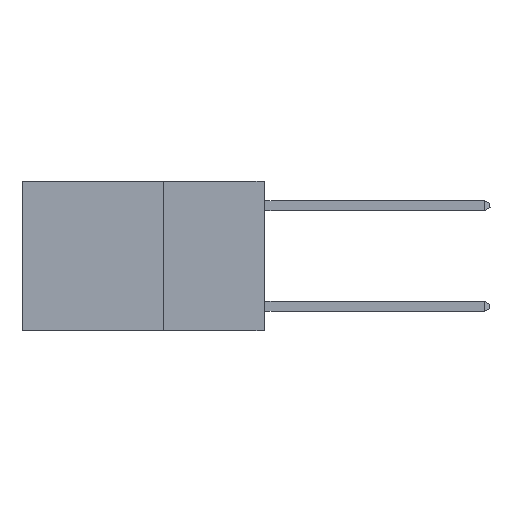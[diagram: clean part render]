
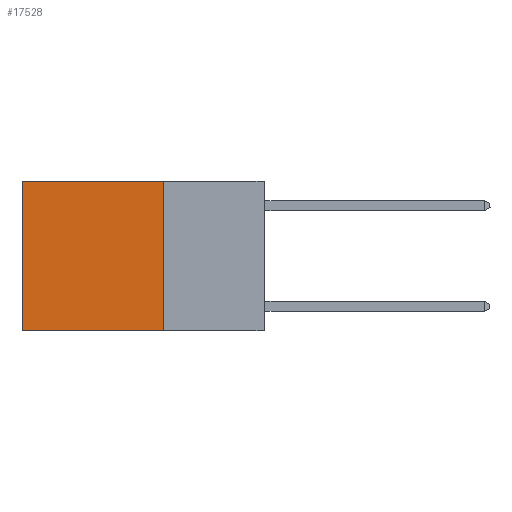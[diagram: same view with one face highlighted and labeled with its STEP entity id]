
A CAD part, left-side view. The second image highlights one B-rep face of the part: STEP entity #17528.
In plain terms, the highlighted planar face has unit normal (-1, 0, 0).
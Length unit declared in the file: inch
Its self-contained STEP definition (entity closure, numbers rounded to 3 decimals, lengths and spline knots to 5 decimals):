
#494 = DIRECTION ( 'NONE',  ( 0., 1., 0. ) ) ;
#1168 = FACE_OUTER_BOUND ( 'NONE', #11827, .T. ) ;
#1943 = EDGE_CURVE ( 'NONE', #18034, #6293, #9952, .T. ) ;
#2007 = CARTESIAN_POINT ( 'NONE',  ( 0.2625, 0.25, 0. ) ) ;
#2605 = DIRECTION ( 'NONE',  ( 1., 0., 0. ) ) ;
#3637 = LINE ( 'NONE', #17984, #12807 ) ;
#5821 = CARTESIAN_POINT ( 'NONE',  ( 0.2625, 0.25, 0. ) ) ;
#6230 = DIRECTION ( 'NONE',  ( 0., 0., -1. ) ) ;
#6293 = VERTEX_POINT ( 'NONE', #15637 ) ;
#7214 = VERTEX_POINT ( 'NONE', #13466 ) ;
#7268 = LINE ( 'NONE', #12769, #22412 ) ;
#9266 = EDGE_CURVE ( 'NONE', #6293, #10761, #21585, .T. ) ;
#9952 = LINE ( 'NONE', #5821, #19855 ) ;
#10431 = ORIENTED_EDGE ( 'NONE', *, *, #9266, .T. ) ;
#10761 = VERTEX_POINT ( 'NONE', #19681 ) ;
#11425 = CARTESIAN_POINT ( 'NONE',  ( 0.2625, 0.25, 0. ) ) ;
#11827 = EDGE_LOOP ( 'NONE', ( #10431, #15646, #11985, #21943 ) ) ;
#11985 = ORIENTED_EDGE ( 'NONE', *, *, #14257, .F. ) ;
#12234 = VECTOR ( 'NONE', #20776, 39.37008 ) ;
#12769 = CARTESIAN_POINT ( 'NONE',  ( 0.2625, 0.25, 0. ) ) ;
#12807 = VECTOR ( 'NONE', #12853, 39.37008 ) ;
#12853 = DIRECTION ( 'NONE',  ( 0., 1., 0. ) ) ;
#13092 = CARTESIAN_POINT ( 'NONE',  ( 0.2625, 0.6, 0. ) ) ;
#13466 = CARTESIAN_POINT ( 'NONE',  ( 0.2625, 0.25, -0.37 ) ) ;
#13933 = EDGE_CURVE ( 'NONE', #7214, #10761, #3637, .T. ) ;
#14257 = EDGE_CURVE ( 'NONE', #18034, #7214, #7268, .T. ) ;
#15108 = DIRECTION ( 'NONE',  ( 0., 0., -1. ) ) ;
#15637 = CARTESIAN_POINT ( 'NONE',  ( 0.2625, 0.6, 0. ) ) ;
#15646 = ORIENTED_EDGE ( 'NONE', *, *, #13933, .F. ) ;
#17528 = ADVANCED_FACE ( 'NONE', ( #1168 ), #22168, .F. ) ;
#17984 = CARTESIAN_POINT ( 'NONE',  ( 0.2625, 0.25, -0.37 ) ) ;
#18034 = VERTEX_POINT ( 'NONE', #2007 ) ;
#19681 = CARTESIAN_POINT ( 'NONE',  ( 0.2625, 0.6, -0.37 ) ) ;
#19855 = VECTOR ( 'NONE', #494, 39.37008 ) ;
#20776 = DIRECTION ( 'NONE',  ( 0., 0., -1. ) ) ;
#21585 = LINE ( 'NONE', #13092, #12234 ) ;
#21943 = ORIENTED_EDGE ( 'NONE', *, *, #1943, .T. ) ;
#22168 = PLANE ( 'NONE',  #22731 ) ;
#22412 = VECTOR ( 'NONE', #15108, 39.37008 ) ;
#22731 = AXIS2_PLACEMENT_3D ( 'NONE', #11425, #2605, #6230 ) ;
